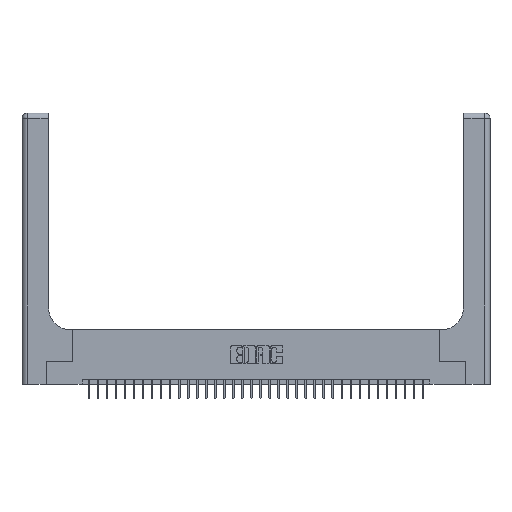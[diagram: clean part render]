
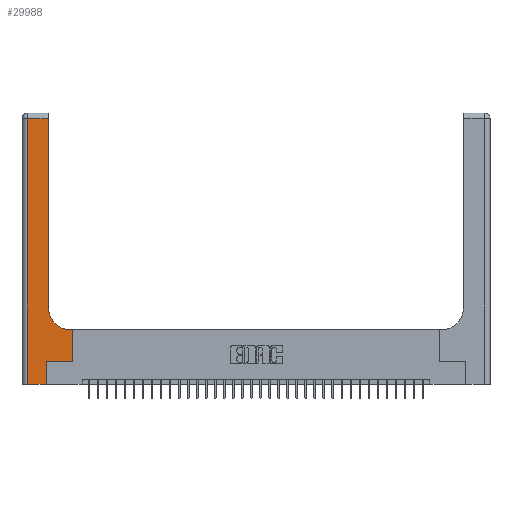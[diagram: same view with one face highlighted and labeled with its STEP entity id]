
A CAD part, top view. The second image highlights one B-rep face of the part: STEP entity #29988.
In plain terms, the highlighted planar face has unit normal (0, 0, 1).
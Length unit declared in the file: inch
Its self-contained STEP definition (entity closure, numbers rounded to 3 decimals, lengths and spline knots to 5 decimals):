
#251 = ORIENTED_EDGE ( 'NONE', *, *, #31819, .T. ) ;
#631 = ORIENTED_EDGE ( 'NONE', *, *, #35522, .T. ) ;
#843 = CARTESIAN_POINT ( 'NONE',  ( 0.06, 2.94, 0.37 ) ) ;
#932 = EDGE_CURVE ( 'NONE', #30668, #14620, #30071, .T. ) ;
#1101 = LINE ( 'NONE', #22473, #13333 ) ;
#2012 = CARTESIAN_POINT ( 'NONE',  ( 0.269, 0.25, 0.37 ) ) ;
#2442 = EDGE_CURVE ( 'NONE', #14620, #10477, #1101, .T. ) ;
#2658 = VERTEX_POINT ( 'NONE', #34026 ) ;
#3399 = EDGE_CURVE ( 'NONE', #34682, #2658, #12153, .T. ) ;
#3704 = PLANE ( 'NONE',  #17568 ) ;
#4135 = ORIENTED_EDGE ( 'NONE', *, *, #15763, .T. ) ;
#4383 = CARTESIAN_POINT ( 'NONE',  ( 0.06, 0., 0.37 ) ) ;
#4385 = LINE ( 'NONE', #2012, #31929 ) ;
#4468 = DIRECTION ( 'NONE',  ( 0., -1., 0. ) ) ;
#4849 = DIRECTION ( 'NONE',  ( 1., 0., 0. ) ) ;
#6514 = EDGE_LOOP ( 'NONE', ( #4135, #29274, #29375, #21757, #16288, #8196, #31693, #251, #631 ) ) ;
#6580 = CARTESIAN_POINT ( 'NONE',  ( 0.5585, 0.25, 0.37 ) ) ;
#7329 = CARTESIAN_POINT ( 'NONE',  ( 0.5415, 0.85, 0.37 ) ) ;
#8196 = ORIENTED_EDGE ( 'NONE', *, *, #19501, .T. ) ;
#8784 = DIRECTION ( 'NONE',  ( 0., 1., 0. ) ) ;
#9277 = VECTOR ( 'NONE', #27343, 39.37008 ) ;
#9352 = DIRECTION ( 'NONE',  ( -1., 0., 0. ) ) ;
#10159 = DIRECTION ( 'NONE',  ( 1., 0., 0. ) ) ;
#10477 = VERTEX_POINT ( 'NONE', #24072 ) ;
#11705 = LINE ( 'NONE', #29474, #19021 ) ;
#11753 = CARTESIAN_POINT ( 'NONE',  ( 0.269, 0.25, 0.37 ) ) ;
#12027 = CARTESIAN_POINT ( 'NONE',  ( 0., 2.94, 0.37 ) ) ;
#12153 = LINE ( 'NONE', #13378, #31384 ) ;
#13333 = VECTOR ( 'NONE', #25190, 39.37008 ) ;
#13378 = CARTESIAN_POINT ( 'NONE',  ( 0.5585, 0.25, 0.37 ) ) ;
#13541 = FACE_OUTER_BOUND ( 'NONE', #6514, .T. ) ;
#13988 = VERTEX_POINT ( 'NONE', #15484 ) ;
#14620 = VERTEX_POINT ( 'NONE', #4383 ) ;
#15484 = CARTESIAN_POINT ( 'NONE',  ( 0.5415, 0.6, 0.37 ) ) ;
#15763 = EDGE_CURVE ( 'NONE', #18261, #29479, #16346, .T. ) ;
#16131 = DIRECTION ( 'NONE',  ( 0., 1., 0. ) ) ;
#16288 = ORIENTED_EDGE ( 'NONE', *, *, #29123, .T. ) ;
#16346 = LINE ( 'NONE', #27985, #23669 ) ;
#16446 = CARTESIAN_POINT ( 'NONE',  ( 0.269, 0., 0.37 ) ) ;
#17568 = AXIS2_PLACEMENT_3D ( 'NONE', #23119, #25833, #9352 ) ;
#18261 = VERTEX_POINT ( 'NONE', #24654 ) ;
#18502 = EDGE_CURVE ( 'NONE', #29479, #30668, #24814, .T. ) ;
#19021 = VECTOR ( 'NONE', #24038, 39.37008 ) ;
#19091 = CIRCLE ( 'NONE', #23687, 0.25 ) ;
#19501 = EDGE_CURVE ( 'NONE', #20921, #34682, #4385, .T. ) ;
#20921 = VERTEX_POINT ( 'NONE', #11753 ) ;
#21610 = CARTESIAN_POINT ( 'NONE',  ( 0.2915, 2.94, 0.37 ) ) ;
#21757 = ORIENTED_EDGE ( 'NONE', *, *, #2442, .T. ) ;
#22473 = CARTESIAN_POINT ( 'NONE',  ( 0., 0., 0.37 ) ) ;
#23119 = CARTESIAN_POINT ( 'NONE',  ( 0., 3., 0.37 ) ) ;
#23669 = VECTOR ( 'NONE', #8784, 39.37008 ) ;
#23687 = AXIS2_PLACEMENT_3D ( 'NONE', #7329, #26615, #10159 ) ;
#24038 = DIRECTION ( 'NONE',  ( -1., 0., 0. ) ) ;
#24072 = CARTESIAN_POINT ( 'NONE',  ( 0.269, 0., 0.37 ) ) ;
#24654 = CARTESIAN_POINT ( 'NONE',  ( 0.2915, 0.85, 0.37 ) ) ;
#24814 = LINE ( 'NONE', #12027, #32000 ) ;
#25190 = DIRECTION ( 'NONE',  ( 1., 0., 0. ) ) ;
#25833 = DIRECTION ( 'NONE',  ( 0., 0., -1. ) ) ;
#26569 = CARTESIAN_POINT ( 'NONE',  ( 0.06, 3., 0.37 ) ) ;
#26615 = DIRECTION ( 'NONE',  ( 0., 0., -1. ) ) ;
#27343 = DIRECTION ( 'NONE',  ( 0., 1., 0. ) ) ;
#27985 = CARTESIAN_POINT ( 'NONE',  ( 0.2915, 3., 0.37 ) ) ;
#29123 = EDGE_CURVE ( 'NONE', #10477, #20921, #31136, .T. ) ;
#29211 = VECTOR ( 'NONE', #4468, 39.37008 ) ;
#29274 = ORIENTED_EDGE ( 'NONE', *, *, #18502, .T. ) ;
#29375 = ORIENTED_EDGE ( 'NONE', *, *, #932, .T. ) ;
#29474 = CARTESIAN_POINT ( 'NONE',  ( 0.2915, 0.6, 0.37 ) ) ;
#29479 = VERTEX_POINT ( 'NONE', #21610 ) ;
#29988 = ADVANCED_FACE ( 'NONE', ( #13541 ), #3704, .F. ) ;
#30071 = LINE ( 'NONE', #26569, #29211 ) ;
#30668 = VERTEX_POINT ( 'NONE', #843 ) ;
#31136 = LINE ( 'NONE', #16446, #9277 ) ;
#31137 = DIRECTION ( 'NONE',  ( -1., 0., 0. ) ) ;
#31384 = VECTOR ( 'NONE', #16131, 39.37008 ) ;
#31693 = ORIENTED_EDGE ( 'NONE', *, *, #3399, .T. ) ;
#31819 = EDGE_CURVE ( 'NONE', #2658, #13988, #11705, .T. ) ;
#31929 = VECTOR ( 'NONE', #4849, 39.37008 ) ;
#32000 = VECTOR ( 'NONE', #31137, 39.37008 ) ;
#34026 = CARTESIAN_POINT ( 'NONE',  ( 0.5585, 0.6, 0.37 ) ) ;
#34682 = VERTEX_POINT ( 'NONE', #6580 ) ;
#35522 = EDGE_CURVE ( 'NONE', #13988, #18261, #19091, .T. ) ;
